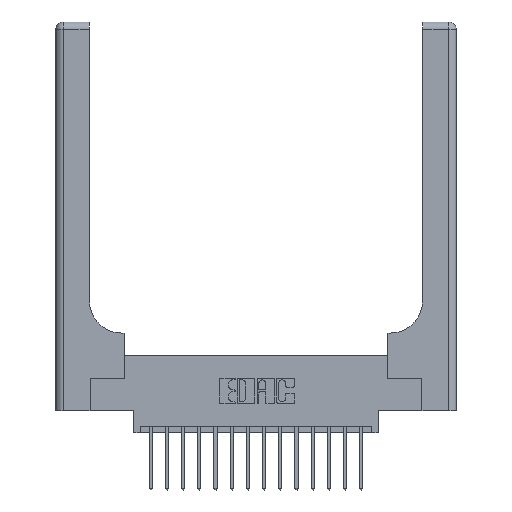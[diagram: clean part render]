
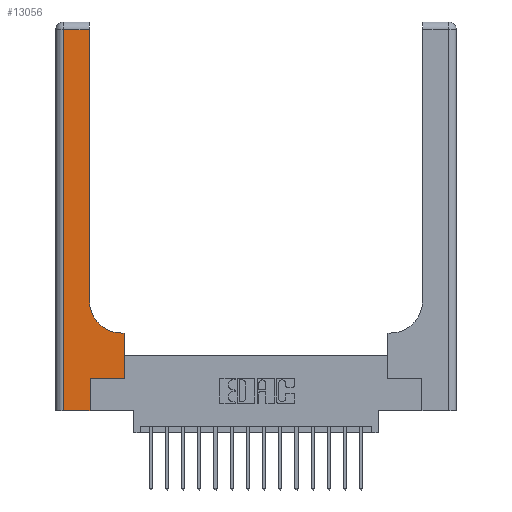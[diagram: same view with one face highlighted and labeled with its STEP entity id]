
A CAD part, top view. The second image highlights one B-rep face of the part: STEP entity #13056.
In plain terms, the highlighted planar face has unit normal (0, 0, 1).
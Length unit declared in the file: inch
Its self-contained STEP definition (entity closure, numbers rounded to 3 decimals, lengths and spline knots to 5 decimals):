
#12 = CARTESIAN_POINT ( 'NONE',  ( 0.528, 0.6, 0.37 ) ) ;
#263 = CARTESIAN_POINT ( 'NONE',  ( 0.26, 2.94, 0.37 ) ) ;
#434 = DIRECTION ( 'NONE',  ( 0., 1., 0. ) ) ;
#1627 = CARTESIAN_POINT ( 'NONE',  ( 0.528, 0.25, 0.37 ) ) ;
#2403 = CIRCLE ( 'NONE', #15366, 0.25 ) ;
#2717 = VECTOR ( 'NONE', #17618, 39.37008 ) ;
#2747 = CARTESIAN_POINT ( 'NONE',  ( 0., 3., 0.37 ) ) ;
#2795 = EDGE_CURVE ( 'NONE', #3301, #5992, #4978, .T. ) ;
#3295 = AXIS2_PLACEMENT_3D ( 'NONE', #2747, #5689, #8339 ) ;
#3301 = VERTEX_POINT ( 'NONE', #3530 ) ;
#3302 = CARTESIAN_POINT ( 'NONE',  ( 0.265, 0., 0.37 ) ) ;
#3324 = LINE ( 'NONE', #4366, #10403 ) ;
#3530 = CARTESIAN_POINT ( 'NONE',  ( 0.26, 0.85, 0.37 ) ) ;
#3633 = ORIENTED_EDGE ( 'NONE', *, *, #6875, .T. ) ;
#3712 = VECTOR ( 'NONE', #434, 39.37008 ) ;
#4313 = DIRECTION ( 'NONE',  ( -1., 0., 0. ) ) ;
#4366 = CARTESIAN_POINT ( 'NONE',  ( 0., 0., 0.37 ) ) ;
#4565 = VERTEX_POINT ( 'NONE', #12 ) ;
#4978 = LINE ( 'NONE', #12234, #3712 ) ;
#5661 = VECTOR ( 'NONE', #16191, 39.37008 ) ;
#5689 = DIRECTION ( 'NONE',  ( 0., 0., -1. ) ) ;
#5732 = CARTESIAN_POINT ( 'NONE',  ( 0.26, 0.6, 0.37 ) ) ;
#5799 = LINE ( 'NONE', #1627, #7281 ) ;
#5836 = DIRECTION ( 'NONE',  ( -1., 0., 0. ) ) ;
#5870 = VERTEX_POINT ( 'NONE', #7359 ) ;
#5992 = VERTEX_POINT ( 'NONE', #263 ) ;
#6102 = CARTESIAN_POINT ( 'NONE',  ( 0.06, 3., 0.37 ) ) ;
#6158 = ORIENTED_EDGE ( 'NONE', *, *, #17014, .T. ) ;
#6294 = ORIENTED_EDGE ( 'NONE', *, *, #12256, .T. ) ;
#6875 = EDGE_CURVE ( 'NONE', #15139, #5870, #3324, .T. ) ;
#7281 = VECTOR ( 'NONE', #13150, 39.37008 ) ;
#7309 = EDGE_CURVE ( 'NONE', #5870, #18542, #17944, .T. ) ;
#7359 = CARTESIAN_POINT ( 'NONE',  ( 0.265, 0., 0.37 ) ) ;
#8339 = DIRECTION ( 'NONE',  ( -1., 0., 0. ) ) ;
#8739 = LINE ( 'NONE', #5732, #10328 ) ;
#9086 = DIRECTION ( 'NONE',  ( 1., 0., 0. ) ) ;
#9277 = EDGE_CURVE ( 'NONE', #18542, #11406, #13539, .T. ) ;
#9489 = ORIENTED_EDGE ( 'NONE', *, *, #16261, .T. ) ;
#10297 = VECTOR ( 'NONE', #5836, 39.37008 ) ;
#10328 = VECTOR ( 'NONE', #4313, 39.37008 ) ;
#10403 = VECTOR ( 'NONE', #9086, 39.37008 ) ;
#10639 = VERTEX_POINT ( 'NONE', #14694 ) ;
#10845 = DIRECTION ( 'NONE',  ( 0., 1., 0. ) ) ;
#11026 = VECTOR ( 'NONE', #10845, 39.37008 ) ;
#11351 = FACE_OUTER_BOUND ( 'NONE', #15698, .T. ) ;
#11406 = VERTEX_POINT ( 'NONE', #12937 ) ;
#11586 = LINE ( 'NONE', #17634, #10297 ) ;
#11783 = PLANE ( 'NONE',  #3295 ) ;
#11849 = LINE ( 'NONE', #6102, #2717 ) ;
#11941 = VERTEX_POINT ( 'NONE', #13100 ) ;
#12234 = CARTESIAN_POINT ( 'NONE',  ( 0.26, 3., 0.37 ) ) ;
#12256 = EDGE_CURVE ( 'NONE', #11941, #3301, #2403, .T. ) ;
#12937 = CARTESIAN_POINT ( 'NONE',  ( 0.528, 0.25, 0.37 ) ) ;
#13056 = ADVANCED_FACE ( 'NONE', ( #11351 ), #11783, .F. ) ;
#13100 = CARTESIAN_POINT ( 'NONE',  ( 0.51, 0.6, 0.37 ) ) ;
#13150 = DIRECTION ( 'NONE',  ( 0., 1., 0. ) ) ;
#13451 = CARTESIAN_POINT ( 'NONE',  ( 0.265, 0.25, 0.37 ) ) ;
#13539 = LINE ( 'NONE', #13451, #5661 ) ;
#14682 = EDGE_CURVE ( 'NONE', #10639, #15139, #11849, .T. ) ;
#14694 = CARTESIAN_POINT ( 'NONE',  ( 0.06, 2.94, 0.37 ) ) ;
#14826 = ORIENTED_EDGE ( 'NONE', *, *, #2795, .T. ) ;
#15139 = VERTEX_POINT ( 'NONE', #17764 ) ;
#15366 = AXIS2_PLACEMENT_3D ( 'NONE', #15817, #17057, #15723 ) ;
#15373 = ORIENTED_EDGE ( 'NONE', *, *, #9277, .T. ) ;
#15698 = EDGE_LOOP ( 'NONE', ( #14826, #18313, #17509, #3633, #15808, #15373, #9489, #6158, #6294 ) ) ;
#15723 = DIRECTION ( 'NONE',  ( 1., 0., 0. ) ) ;
#15808 = ORIENTED_EDGE ( 'NONE', *, *, #7309, .T. ) ;
#15817 = CARTESIAN_POINT ( 'NONE',  ( 0.51, 0.85, 0.37 ) ) ;
#16191 = DIRECTION ( 'NONE',  ( 1., 0., 0. ) ) ;
#16261 = EDGE_CURVE ( 'NONE', #11406, #4565, #5799, .T. ) ;
#17014 = EDGE_CURVE ( 'NONE', #4565, #11941, #8739, .T. ) ;
#17057 = DIRECTION ( 'NONE',  ( 0., 0., -1. ) ) ;
#17509 = ORIENTED_EDGE ( 'NONE', *, *, #14682, .T. ) ;
#17583 = EDGE_CURVE ( 'NONE', #5992, #10639, #11586, .T. ) ;
#17618 = DIRECTION ( 'NONE',  ( 0., -1., 0. ) ) ;
#17634 = CARTESIAN_POINT ( 'NONE',  ( 0., 2.94, 0.37 ) ) ;
#17764 = CARTESIAN_POINT ( 'NONE',  ( 0.06, 0., 0.37 ) ) ;
#17944 = LINE ( 'NONE', #3302, #11026 ) ;
#18313 = ORIENTED_EDGE ( 'NONE', *, *, #17583, .T. ) ;
#18507 = CARTESIAN_POINT ( 'NONE',  ( 0.265, 0.25, 0.37 ) ) ;
#18542 = VERTEX_POINT ( 'NONE', #18507 ) ;
